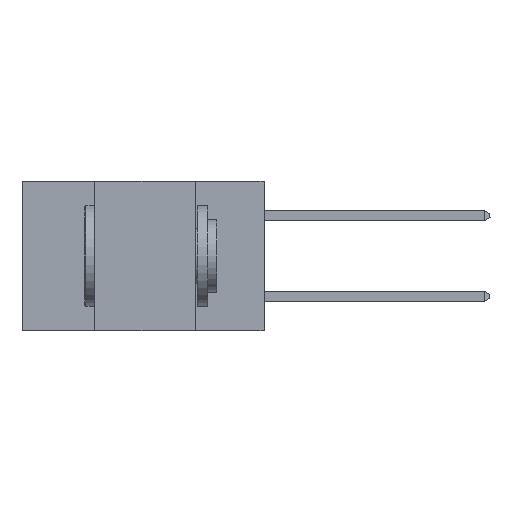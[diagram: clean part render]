
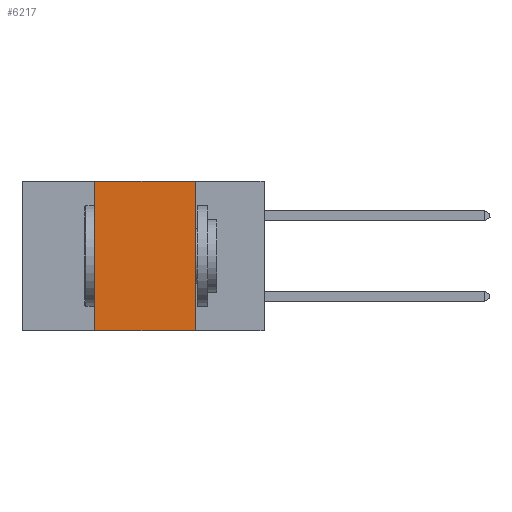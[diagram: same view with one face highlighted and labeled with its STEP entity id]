
A CAD part, left-side view. The second image highlights one B-rep face of the part: STEP entity #6217.
In plain terms, the highlighted planar face has unit normal (-1, 0, 0).
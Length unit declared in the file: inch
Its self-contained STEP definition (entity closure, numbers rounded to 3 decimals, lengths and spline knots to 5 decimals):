
#993 = VERTEX_POINT ( 'NONE', #5750 ) ;
#1229 = FACE_OUTER_BOUND ( 'NONE', #11920, .T. ) ;
#1235 = ORIENTED_EDGE ( 'NONE', *, *, #5447, .F. ) ;
#1251 = ORIENTED_EDGE ( 'NONE', *, *, #11768, .T. ) ;
#1562 = LINE ( 'NONE', #4879, #8721 ) ;
#2142 = DIRECTION ( 'NONE',  ( 0., -1., 0. ) ) ;
#3127 = CARTESIAN_POINT ( 'NONE',  ( 0., 0.17, 0. ) ) ;
#3524 = ORIENTED_EDGE ( 'NONE', *, *, #4035, .F. ) ;
#4035 = EDGE_CURVE ( 'NONE', #993, #10218, #6807, .T. ) ;
#4584 = CARTESIAN_POINT ( 'NONE',  ( 0., 0.17, 0. ) ) ;
#4813 = VERTEX_POINT ( 'NONE', #10993 ) ;
#4879 = CARTESIAN_POINT ( 'NONE',  ( 0., 0.6, 0. ) ) ;
#5030 = VECTOR ( 'NONE', #12035, 39.37008 ) ;
#5067 = VECTOR ( 'NONE', #9149, 39.37008 ) ;
#5212 = EDGE_CURVE ( 'NONE', #10218, #11469, #1562, .T. ) ;
#5447 = EDGE_CURVE ( 'NONE', #11469, #4813, #10584, .T. ) ;
#5750 = CARTESIAN_POINT ( 'NONE',  ( 0., 0.42, -0.37 ) ) ;
#5920 = DIRECTION ( 'NONE',  ( 0., -1., 0. ) ) ;
#6217 = ADVANCED_FACE ( 'NONE', ( #1229 ), #8536, .F. ) ;
#6280 = CARTESIAN_POINT ( 'NONE',  ( 0., 0.42, 0. ) ) ;
#6329 = LINE ( 'NONE', #11524, #10004 ) ;
#6807 = LINE ( 'NONE', #6280, #5067 ) ;
#7770 = AXIS2_PLACEMENT_3D ( 'NONE', #9433, #11356, #8580 ) ;
#8536 = PLANE ( 'NONE',  #7770 ) ;
#8580 = DIRECTION ( 'NONE',  ( 0., 0., -1. ) ) ;
#8721 = VECTOR ( 'NONE', #2142, 39.37008 ) ;
#9149 = DIRECTION ( 'NONE',  ( 0., 0., 1. ) ) ;
#9433 = CARTESIAN_POINT ( 'NONE',  ( 0., 0.6, 0. ) ) ;
#10004 = VECTOR ( 'NONE', #5920, 39.37008 ) ;
#10218 = VERTEX_POINT ( 'NONE', #10855 ) ;
#10584 = LINE ( 'NONE', #4584, #5030 ) ;
#10855 = CARTESIAN_POINT ( 'NONE',  ( 0., 0.42, 0. ) ) ;
#10993 = CARTESIAN_POINT ( 'NONE',  ( 0., 0.17, -0.37 ) ) ;
#11036 = ORIENTED_EDGE ( 'NONE', *, *, #5212, .F. ) ;
#11356 = DIRECTION ( 'NONE',  ( 1., 0., 0. ) ) ;
#11469 = VERTEX_POINT ( 'NONE', #3127 ) ;
#11524 = CARTESIAN_POINT ( 'NONE',  ( 0., 0.6, -0.37 ) ) ;
#11768 = EDGE_CURVE ( 'NONE', #993, #4813, #6329, .T. ) ;
#11920 = EDGE_LOOP ( 'NONE', ( #1235, #11036, #3524, #1251 ) ) ;
#12035 = DIRECTION ( 'NONE',  ( 0., 0., -1. ) ) ;
